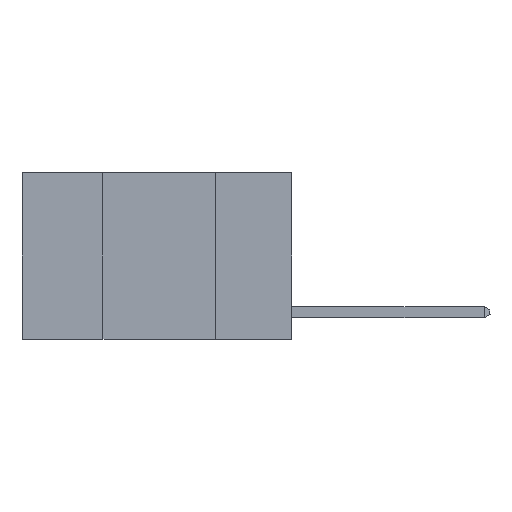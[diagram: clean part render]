
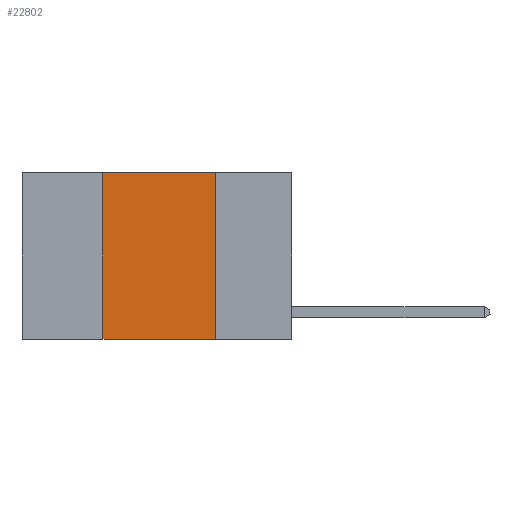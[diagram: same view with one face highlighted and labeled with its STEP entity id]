
A CAD part, left-side view. The second image highlights one B-rep face of the part: STEP entity #22802.
In plain terms, the highlighted planar face has unit normal (-1, 0, 0).
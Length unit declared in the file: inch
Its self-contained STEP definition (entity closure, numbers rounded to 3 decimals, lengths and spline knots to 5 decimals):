
#1095 = DIRECTION ( 'NONE',  ( 0., 0., -1. ) ) ;
#1412 = EDGE_CURVE ( 'NONE', #10851, #10811, #19364, .T. ) ;
#2277 = VECTOR ( 'NONE', #8286, 39.37008 ) ;
#2541 = FACE_OUTER_BOUND ( 'NONE', #5135, .T. ) ;
#3323 = DIRECTION ( 'NONE',  ( 0., -1., 0. ) ) ;
#4433 = PLANE ( 'NONE',  #22755 ) ;
#4491 = LINE ( 'NONE', #14165, #27030 ) ;
#5135 = EDGE_LOOP ( 'NONE', ( #8483, #9246, #12639, #23904 ) ) ;
#5239 = DIRECTION ( 'NONE',  ( 0., -1., 0. ) ) ;
#6105 = CARTESIAN_POINT ( 'NONE',  ( 0., 0.42, 0. ) ) ;
#6460 = VERTEX_POINT ( 'NONE', #12297 ) ;
#6576 = VECTOR ( 'NONE', #5239, 39.37008 ) ;
#6684 = DIRECTION ( 'NONE',  ( 1., 0., 0. ) ) ;
#7256 = CARTESIAN_POINT ( 'NONE',  ( 0., 0.42, -0.37 ) ) ;
#8286 = DIRECTION ( 'NONE',  ( 0., 0., 1. ) ) ;
#8483 = ORIENTED_EDGE ( 'NONE', *, *, #1412, .F. ) ;
#8789 = CARTESIAN_POINT ( 'NONE',  ( 0., 0.6, 0. ) ) ;
#9246 = ORIENTED_EDGE ( 'NONE', *, *, #19463, .F. ) ;
#10811 = VERTEX_POINT ( 'NONE', #12118 ) ;
#10851 = VERTEX_POINT ( 'NONE', #27544 ) ;
#12118 = CARTESIAN_POINT ( 'NONE',  ( 0., 0.17, -0.37 ) ) ;
#12297 = CARTESIAN_POINT ( 'NONE',  ( 0., 0.42, 0. ) ) ;
#12357 = LINE ( 'NONE', #13927, #6576 ) ;
#12639 = ORIENTED_EDGE ( 'NONE', *, *, #21321, .F. ) ;
#13526 = VECTOR ( 'NONE', #1095, 39.37008 ) ;
#13927 = CARTESIAN_POINT ( 'NONE',  ( 0., 0.6, -0.37 ) ) ;
#14165 = CARTESIAN_POINT ( 'NONE',  ( 0., 0.6, 0. ) ) ;
#14760 = VERTEX_POINT ( 'NONE', #7256 ) ;
#19364 = LINE ( 'NONE', #25181, #13526 ) ;
#19463 = EDGE_CURVE ( 'NONE', #6460, #10851, #4491, .T. ) ;
#21321 = EDGE_CURVE ( 'NONE', #14760, #6460, #24914, .T. ) ;
#21942 = DIRECTION ( 'NONE',  ( 0., 0., -1. ) ) ;
#22755 = AXIS2_PLACEMENT_3D ( 'NONE', #8789, #6684, #21942 ) ;
#22802 = ADVANCED_FACE ( 'NONE', ( #2541 ), #4433, .F. ) ;
#23904 = ORIENTED_EDGE ( 'NONE', *, *, #25835, .T. ) ;
#24914 = LINE ( 'NONE', #6105, #2277 ) ;
#25181 = CARTESIAN_POINT ( 'NONE',  ( 0., 0.17, 0. ) ) ;
#25835 = EDGE_CURVE ( 'NONE', #14760, #10811, #12357, .T. ) ;
#27030 = VECTOR ( 'NONE', #3323, 39.37008 ) ;
#27544 = CARTESIAN_POINT ( 'NONE',  ( 0., 0.17, 0. ) ) ;
